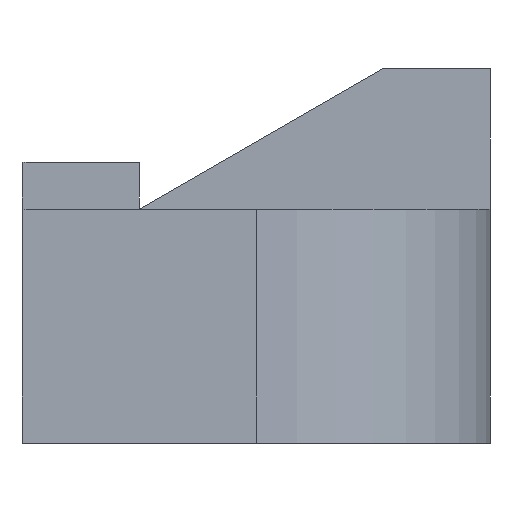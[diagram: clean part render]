
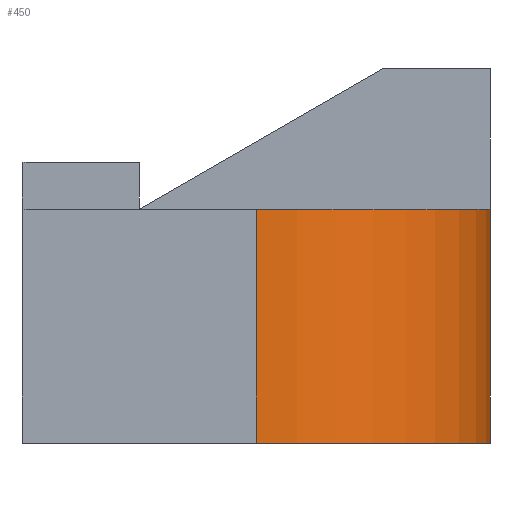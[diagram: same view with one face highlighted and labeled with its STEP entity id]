
A CAD part, front view. The second image highlights one B-rep face of the part: STEP entity #450.
In plain terms, the highlighted cylindrical face has radius 5 mm (diameter 10 mm), a partial arc.
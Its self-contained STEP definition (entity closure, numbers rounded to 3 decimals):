
#390=CARTESIAN_POINT('',(10.,5.,0.0));
#391=VERTEX_POINT('',#390);
#401=CARTESIAN_POINT('',(10.,5.,5.0));
#402=VERTEX_POINT('',#401);
#409=CARTESIAN_POINT('',(10.,5.,0.0));
#410=DIRECTION('',(0.0,0.0,1.0));
#411=VECTOR('',#410,5.0);
#412=LINE('',#409,#411);
#413=EDGE_CURVE('',#391,#402,#412,.T.);
#418=CARTESIAN_POINT('',(5.,5.0,0.0));
#419=DIRECTION('',(0.0,0.0,1.0));
#420=DIRECTION('',(0.0,1.0,0.0));
#421=AXIS2_PLACEMENT_3D('',#418,#419,#420);
#422=CYLINDRICAL_SURFACE('',#421,5.0);
#423=CARTESIAN_POINT('',(5.,0.0,0.0));
#424=VERTEX_POINT('',#423);
#425=CARTESIAN_POINT('',(5.,5.0,0.0));
#426=DIRECTION('',(0.0,0.0,-1.0));
#427=DIRECTION('',(0.0,1.0,0.0));
#428=AXIS2_PLACEMENT_3D('',#425,#426,#427);
#429=CIRCLE('',#428,5.0);
#430=EDGE_CURVE('',#391,#424,#429,.T.);
#431=ORIENTED_EDGE('',*,*,#430,.F.);
#432=ORIENTED_EDGE('',*,*,#413,.T.);
#433=CARTESIAN_POINT('',(5.,0.0,5.0));
#434=VERTEX_POINT('',#433);
#435=CARTESIAN_POINT('',(5.,5.0,5.0));
#436=DIRECTION('',(0.0,0.0,1.0));
#437=DIRECTION('',(0.0,1.0,0.0));
#438=AXIS2_PLACEMENT_3D('',#435,#436,#437);
#439=CIRCLE('',#438,5.0);
#440=EDGE_CURVE('',#434,#402,#439,.T.);
#441=ORIENTED_EDGE('',*,*,#440,.F.);
#442=CARTESIAN_POINT('',(5.,0.0,0.0));
#443=DIRECTION('',(0.0,0.0,1.0));
#444=VECTOR('',#443,5.0);
#445=LINE('',#442,#444);
#446=EDGE_CURVE('',#424,#434,#445,.T.);
#447=ORIENTED_EDGE('',*,*,#446,.F.);
#448=EDGE_LOOP('',(#431,#432,#441,#447));
#449=FACE_OUTER_BOUND('',#448,.T.);
#450=ADVANCED_FACE('',(#449),#422,.T.);
